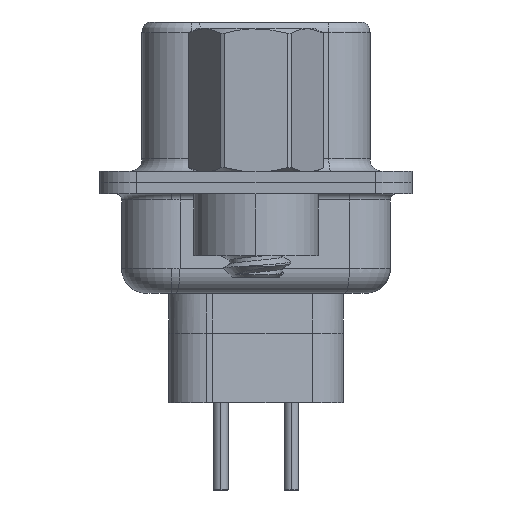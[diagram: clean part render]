
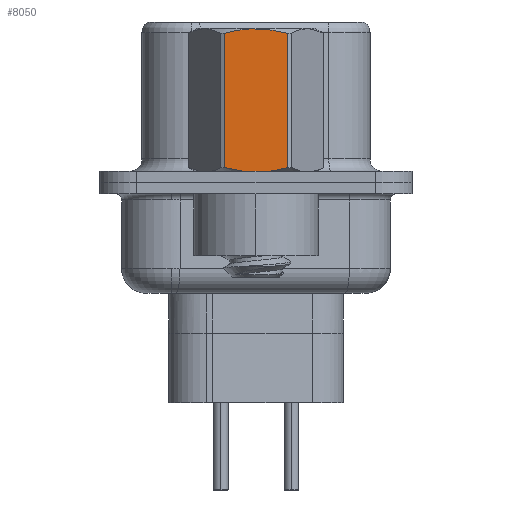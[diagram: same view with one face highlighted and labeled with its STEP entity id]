
A CAD part, left-side view. The second image highlights one B-rep face of the part: STEP entity #8050.
In plain terms, the highlighted planar face has unit normal (-1, 0, 0).
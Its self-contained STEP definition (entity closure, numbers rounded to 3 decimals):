
#416 = CARTESIAN_POINT ( 'NONE',  ( -2.381, 0.853, 6.101 ) ) ;
#907 = CARTESIAN_POINT ( 'NONE',  ( -2.381, 0.428, 6.165 ) ) ;
#1844 = ORIENTED_EDGE ( 'NONE', *, *, #4510, .T. ) ;
#2616 = LINE ( 'NONE', #3246, #13178 ) ;
#3192 = CARTESIAN_POINT ( 'NONE',  ( -2.381, -1.066, 0.546 ) ) ;
#3246 = CARTESIAN_POINT ( 'NONE',  ( -2.381, -1.273, 3.792 ) ) ;
#3468 = CARTESIAN_POINT ( 'NONE',  ( -2.381, -0.215, 6.182 ) ) ;
#4510 = EDGE_CURVE ( 'NONE', #7112, #29221, #2616, .T. ) ;
#5146 = CARTESIAN_POINT ( 'NONE',  ( -2.381, 0.853, 0.499 ) ) ;
#5434 = CARTESIAN_POINT ( 'NONE',  ( -2.381, 1.273, 5.998 ) ) ;
#6458 = CARTESIAN_POINT ( 'NONE',  ( -2.381, 1.273, 5.998 ) ) ;
#7112 = VERTEX_POINT ( 'NONE', #26429 ) ;
#7135 = FACE_OUTER_BOUND ( 'NONE', #12794, .T. ) ;
#7391 = CARTESIAN_POINT ( 'NONE',  ( -2.381, -0.215, 0.418 ) ) ;
#7682 = VERTEX_POINT ( 'NONE', #28809 ) ;
#7823 = CARTESIAN_POINT ( 'NONE',  ( -2.381, -1.273, 5.998 ) ) ;
#8050 = ADVANCED_FACE ( 'NONE', ( #7135 ), #26512, .T. ) ;
#8143 = CARTESIAN_POINT ( 'NONE',  ( -2.381, -0.432, 6.165 ) ) ;
#8556 = EDGE_CURVE ( 'NONE', #22616, #7682, #14313, .T. ) ;
#9550 = DIRECTION ( 'NONE',  ( -1., 0., 0. ) ) ;
#9979 = ORIENTED_EDGE ( 'NONE', *, *, #10542, .T. ) ;
#10238 = CARTESIAN_POINT ( 'NONE',  ( -2.381, 1.065, 6.054 ) ) ;
#10542 = EDGE_CURVE ( 'NONE', #7682, #7112, #27204, .T. ) ;
#11871 = B_SPLINE_CURVE_WITH_KNOTS ( 'NONE', 3,
 ( #7823, #30087, #15683, #8143, #3468, #15515, #907, #416, #10238, #5434 ),
 .UNSPECIFIED., .F., .F.,
 ( 4, 2, 2, 2, 4 ),
 ( 0.001, 0.002, 0.002, 0.003, 0.004 ),
 .UNSPECIFIED. ) ;
#12794 = EDGE_LOOP ( 'NONE', ( #9979, #1844, #31077, #15157 ) ) ;
#13178 = VECTOR ( 'NONE', #27315, 1000. ) ;
#14313 = LINE ( 'NONE', #16396, #23891 ) ;
#15157 = ORIENTED_EDGE ( 'NONE', *, *, #8556, .T. ) ;
#15515 = CARTESIAN_POINT ( 'NONE',  ( -2.381, 0.215, 6.182 ) ) ;
#15683 = CARTESIAN_POINT ( 'NONE',  ( -2.381, -0.858, 6.1 ) ) ;
#16396 = CARTESIAN_POINT ( 'NONE',  ( -2.381, 1.273, 3.792 ) ) ;
#16562 = DIRECTION ( 'NONE',  ( 0., 0., -1. ) ) ;
#17242 = CARTESIAN_POINT ( 'NONE',  ( -2.381, 1.375, -3.8 ) ) ;
#17639 = CARTESIAN_POINT ( 'NONE',  ( -2.381, 1.065, 0.546 ) ) ;
#20189 = CARTESIAN_POINT ( 'NONE',  ( -2.381, 0.428, 0.435 ) ) ;
#22616 = VERTEX_POINT ( 'NONE', #6458 ) ;
#23891 = VECTOR ( 'NONE', #16562, 1000. ) ;
#25156 = CARTESIAN_POINT ( 'NONE',  ( -2.381, 0.215, 0.418 ) ) ;
#25908 = AXIS2_PLACEMENT_3D ( 'NONE', #17242, #9550, #29248 ) ;
#26429 = CARTESIAN_POINT ( 'NONE',  ( -2.381, -1.273, 0.602 ) ) ;
#26512 = PLANE ( 'NONE',  #25908 ) ;
#27055 = EDGE_CURVE ( 'NONE', #29221, #22616, #11871, .T. ) ;
#27204 = B_SPLINE_CURVE_WITH_KNOTS ( 'NONE', 3,
 ( #29339, #17639, #5146, #20189, #25156, #7391, #27412, #29652, #3192, #29811 ),
 .UNSPECIFIED., .F., .F.,
 ( 4, 2, 2, 2, 4 ),
 ( 0.003, 0.003, 0.004, 0.004, 0.005 ),
 .UNSPECIFIED. ) ;
#27315 = DIRECTION ( 'NONE',  ( 0., 0., 1. ) ) ;
#27412 = CARTESIAN_POINT ( 'NONE',  ( -2.381, -0.432, 0.435 ) ) ;
#28809 = CARTESIAN_POINT ( 'NONE',  ( -2.381, 1.273, 0.602 ) ) ;
#29221 = VERTEX_POINT ( 'NONE', #29554 ) ;
#29248 = DIRECTION ( 'NONE',  ( 0., -1., 0. ) ) ;
#29339 = CARTESIAN_POINT ( 'NONE',  ( -2.381, 1.273, 0.602 ) ) ;
#29554 = CARTESIAN_POINT ( 'NONE',  ( -2.381, -1.273, 5.998 ) ) ;
#29652 = CARTESIAN_POINT ( 'NONE',  ( -2.381, -0.858, 0.5 ) ) ;
#29811 = CARTESIAN_POINT ( 'NONE',  ( -2.381, -1.273, 0.602 ) ) ;
#30087 = CARTESIAN_POINT ( 'NONE',  ( -2.381, -1.066, 6.054 ) ) ;
#31077 = ORIENTED_EDGE ( 'NONE', *, *, #27055, .T. ) ;
